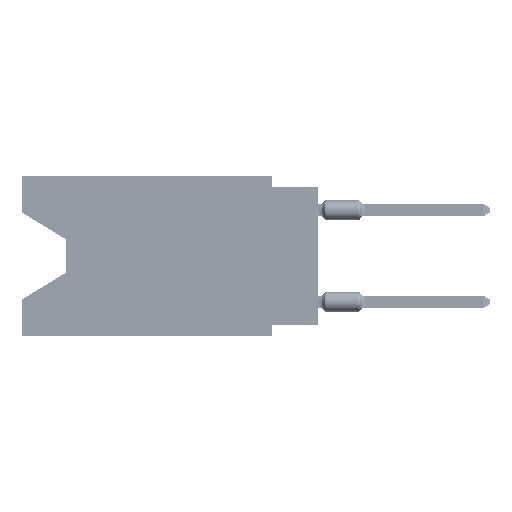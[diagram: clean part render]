
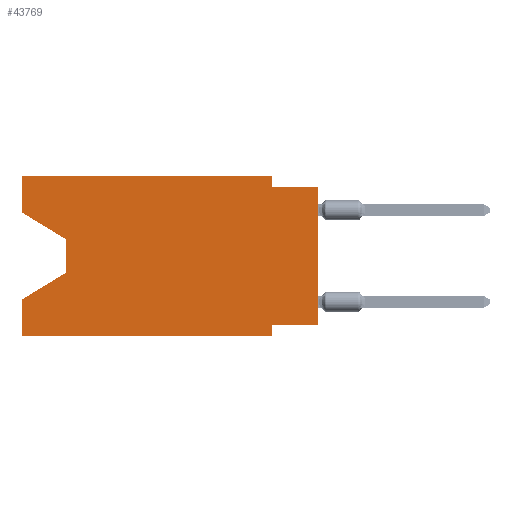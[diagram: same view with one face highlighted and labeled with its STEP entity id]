
A CAD part, left-side view. The second image highlights one B-rep face of the part: STEP entity #43769.
In plain terms, the highlighted planar face has unit normal (-1, 0, 0).
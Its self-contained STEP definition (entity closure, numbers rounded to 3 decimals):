
#841 = EDGE_LOOP ( 'NONE', ( #6417, #49265, #18799, #17559, #33927, #41388, #28121, #76227, #60257, #23435, #69182, #39990 ) ) ;
#1136 = VECTOR ( 'NONE', #74494, 1000. ) ;
#1149 = VECTOR ( 'NONE', #75870, 1000. ) ;
#2669 = EDGE_CURVE ( 'NONE', #33955, #25655, #46566, .T. ) ;
#3153 = VERTEX_POINT ( 'NONE', #48767 ) ;
#4778 = EDGE_CURVE ( 'NONE', #33916, #11526, #58924, .T. ) ;
#5416 = FACE_OUTER_BOUND ( 'NONE', #841, .T. ) ;
#6188 = DIRECTION ( 'NONE',  ( 0., 0., -1. ) ) ;
#6417 = ORIENTED_EDGE ( 'NONE', *, *, #59963, .T. ) ;
#6584 = CARTESIAN_POINT ( 'NONE',  ( 0., 16.383, -8.89 ) ) ;
#6664 = LINE ( 'NONE', #55253, #52635 ) ;
#8201 = EDGE_CURVE ( 'NONE', #25655, #63633, #8325, .T. ) ;
#8325 = LINE ( 'NONE', #71043, #54166 ) ;
#11526 = VERTEX_POINT ( 'NONE', #46878 ) ;
#12443 = CARTESIAN_POINT ( 'NONE',  ( 0., 16.383, -6.852 ) ) ;
#12566 = CARTESIAN_POINT ( 'NONE',  ( 0., 16.383, 0. ) ) ;
#12870 = AXIS2_PLACEMENT_3D ( 'NONE', #61661, #41858, #6188 ) ;
#13053 = EDGE_CURVE ( 'NONE', #31189, #3153, #19713, .T. ) ;
#17559 = ORIENTED_EDGE ( 'NONE', *, *, #44268, .F. ) ;
#17691 = VERTEX_POINT ( 'NONE', #64299 ) ;
#17789 = EDGE_CURVE ( 'NONE', #31189, #73107, #6664, .T. ) ;
#18104 = LINE ( 'NONE', #36736, #34868 ) ;
#18799 = ORIENTED_EDGE ( 'NONE', *, *, #8201, .T. ) ;
#19713 = LINE ( 'NONE', #26574, #37065 ) ;
#20698 = CARTESIAN_POINT ( 'NONE',  ( 0., 16.383, -8.89 ) ) ;
#21266 = VERTEX_POINT ( 'NONE', #20698 ) ;
#23435 = ORIENTED_EDGE ( 'NONE', *, *, #72478, .F. ) ;
#25121 = LINE ( 'NONE', #12566, #1136 ) ;
#25655 = VERTEX_POINT ( 'NONE', #66313 ) ;
#26574 = CARTESIAN_POINT ( 'NONE',  ( 0., 0., 0. ) ) ;
#26777 = LINE ( 'NONE', #6584, #32108 ) ;
#28121 = ORIENTED_EDGE ( 'NONE', *, *, #17789, .F. ) ;
#28683 = CARTESIAN_POINT ( 'NONE',  ( 0., 16.383, -2.038 ) ) ;
#28937 = CARTESIAN_POINT ( 'NONE',  ( 0., 16.383, 0. ) ) ;
#28974 = CARTESIAN_POINT ( 'NONE',  ( 0., 16.383, -2.038 ) ) ;
#29674 = VECTOR ( 'NONE', #71531, 1000. ) ;
#31189 = VERTEX_POINT ( 'NONE', #62921 ) ;
#32108 = VECTOR ( 'NONE', #50709, 1000. ) ;
#32837 = EDGE_CURVE ( 'NONE', #21266, #49341, #26777, .T. ) ;
#33916 = VERTEX_POINT ( 'NONE', #28974 ) ;
#33927 = ORIENTED_EDGE ( 'NONE', *, *, #32837, .T. ) ;
#33955 = VERTEX_POINT ( 'NONE', #53156 ) ;
#34449 = VERTEX_POINT ( 'NONE', #45367 ) ;
#34547 = LINE ( 'NONE', #45926, #1149 ) ;
#34868 = VECTOR ( 'NONE', #54563, 1000. ) ;
#35066 = CARTESIAN_POINT ( 'NONE',  ( 0., 2.54, -8.89 ) ) ;
#35809 = DIRECTION ( 'NONE',  ( 0., 0., 1. ) ) ;
#36736 = CARTESIAN_POINT ( 'NONE',  ( 0., 2.54, -8.89 ) ) ;
#36974 = PLANE ( 'NONE',  #12870 ) ;
#37065 = VECTOR ( 'NONE', #52078, 1000. ) ;
#38564 = EDGE_CURVE ( 'NONE', #11526, #17691, #60176, .T. ) ;
#39889 = DIRECTION ( 'NONE',  ( 0., 0.855, -0.519 ) ) ;
#39990 = ORIENTED_EDGE ( 'NONE', *, *, #4778, .F. ) ;
#41388 = ORIENTED_EDGE ( 'NONE', *, *, #70811, .F. ) ;
#41858 = DIRECTION ( 'NONE',  ( 1., 0., 0. ) ) ;
#43769 = ADVANCED_FACE ( 'NONE', ( #5416 ), #36974, .F. ) ;
#44268 = EDGE_CURVE ( 'NONE', #21266, #63633, #25121, .T. ) ;
#45367 = CARTESIAN_POINT ( 'NONE',  ( 0., 2.54, -0.635 ) ) ;
#45926 = CARTESIAN_POINT ( 'NONE',  ( 0., 0., -0.635 ) ) ;
#46566 = LINE ( 'NONE', #65182, #47111 ) ;
#46878 = CARTESIAN_POINT ( 'NONE',  ( 0., 16.383, 0. ) ) ;
#46896 = DIRECTION ( 'NONE',  ( 0., 1., 0. ) ) ;
#46929 = DIRECTION ( 'NONE',  ( 0., -0.855, -0.519 ) ) ;
#47111 = VECTOR ( 'NONE', #71243, 1000. ) ;
#48767 = CARTESIAN_POINT ( 'NONE',  ( 0., 0., -0.635 ) ) ;
#49265 = ORIENTED_EDGE ( 'NONE', *, *, #2669, .T. ) ;
#49341 = VERTEX_POINT ( 'NONE', #35066 ) ;
#50614 = VECTOR ( 'NONE', #55680, 1000. ) ;
#50709 = DIRECTION ( 'NONE',  ( 0., -1., 0. ) ) ;
#52078 = DIRECTION ( 'NONE',  ( 0., 0., 1. ) ) ;
#52635 = VECTOR ( 'NONE', #46896, 1000. ) ;
#53156 = CARTESIAN_POINT ( 'NONE',  ( 0., 13.97, -3.505 ) ) ;
#54166 = VECTOR ( 'NONE', #39889, 1000. ) ;
#54563 = DIRECTION ( 'NONE',  ( 0., 0., -1. ) ) ;
#55253 = CARTESIAN_POINT ( 'NONE',  ( 0., 0., -8.255 ) ) ;
#55680 = DIRECTION ( 'NONE',  ( 0., 0., -1. ) ) ;
#57503 = VECTOR ( 'NONE', #35809, 1000. ) ;
#58924 = LINE ( 'NONE', #28937, #57503 ) ;
#59963 = EDGE_CURVE ( 'NONE', #33916, #33955, #66331, .T. ) ;
#60176 = LINE ( 'NONE', #65852, #29674 ) ;
#60257 = ORIENTED_EDGE ( 'NONE', *, *, #64435, .F. ) ;
#61661 = CARTESIAN_POINT ( 'NONE',  ( 0., 16.383, 0. ) ) ;
#61738 = CARTESIAN_POINT ( 'NONE',  ( 0., 2.54, 0. ) ) ;
#62921 = CARTESIAN_POINT ( 'NONE',  ( 0., 0., -8.255 ) ) ;
#63633 = VERTEX_POINT ( 'NONE', #12443 ) ;
#64299 = CARTESIAN_POINT ( 'NONE',  ( 0., 2.54, 0. ) ) ;
#64435 = EDGE_CURVE ( 'NONE', #34449, #3153, #34547, .T. ) ;
#65182 = CARTESIAN_POINT ( 'NONE',  ( 0., 13.97, -3.505 ) ) ;
#65852 = CARTESIAN_POINT ( 'NONE',  ( 0., 16.383, 0. ) ) ;
#66313 = CARTESIAN_POINT ( 'NONE',  ( 0., 13.97, -5.385 ) ) ;
#66331 = LINE ( 'NONE', #28683, #75810 ) ;
#67012 = LINE ( 'NONE', #61738, #50614 ) ;
#69182 = ORIENTED_EDGE ( 'NONE', *, *, #38564, .F. ) ;
#70811 = EDGE_CURVE ( 'NONE', #73107, #49341, #18104, .T. ) ;
#71043 = CARTESIAN_POINT ( 'NONE',  ( 0., 13.97, -5.385 ) ) ;
#71243 = DIRECTION ( 'NONE',  ( 0., 0., -1. ) ) ;
#71300 = CARTESIAN_POINT ( 'NONE',  ( 0., 2.54, -8.255 ) ) ;
#71531 = DIRECTION ( 'NONE',  ( 0., -1., 0. ) ) ;
#72478 = EDGE_CURVE ( 'NONE', #17691, #34449, #67012, .T. ) ;
#73107 = VERTEX_POINT ( 'NONE', #71300 ) ;
#74494 = DIRECTION ( 'NONE',  ( 0., 0., 1. ) ) ;
#75810 = VECTOR ( 'NONE', #46929, 1000. ) ;
#75870 = DIRECTION ( 'NONE',  ( 0., -1., 0. ) ) ;
#76227 = ORIENTED_EDGE ( 'NONE', *, *, #13053, .T. ) ;
